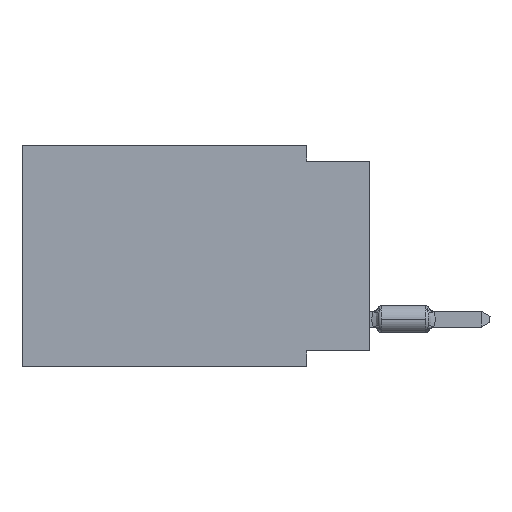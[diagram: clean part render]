
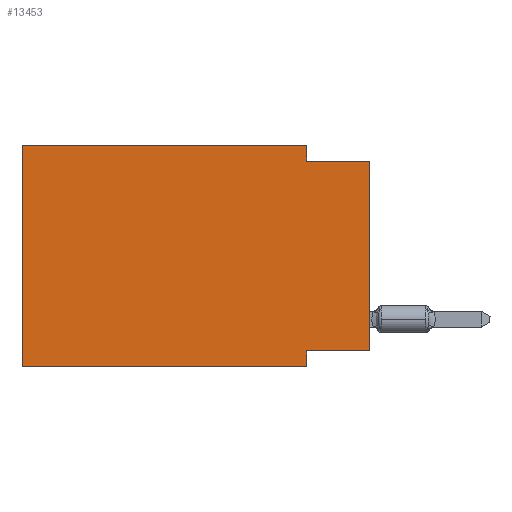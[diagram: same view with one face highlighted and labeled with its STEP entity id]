
A CAD part, left-side view. The second image highlights one B-rep face of the part: STEP entity #13453.
In plain terms, the highlighted planar face has unit normal (-1, 0, 0).
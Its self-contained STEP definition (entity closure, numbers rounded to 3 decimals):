
#489 = VERTEX_POINT ( 'NONE', #13293 ) ;
#593 = CARTESIAN_POINT ( 'NONE',  ( 0., 0., -8.255 ) ) ;
#1355 = VERTEX_POINT ( 'NONE', #31852 ) ;
#1724 = ORIENTED_EDGE ( 'NONE', *, *, #13110, .F. ) ;
#1796 = VECTOR ( 'NONE', #28328, 1000. ) ;
#2309 = ORIENTED_EDGE ( 'NONE', *, *, #19453, .T. ) ;
#2526 = EDGE_CURVE ( 'NONE', #1355, #23772, #24525, .T. ) ;
#3604 = ORIENTED_EDGE ( 'NONE', *, *, #8914, .F. ) ;
#4480 = VERTEX_POINT ( 'NONE', #32439 ) ;
#5051 = CARTESIAN_POINT ( 'NONE',  ( 0., 2.54, 0. ) ) ;
#7102 = EDGE_CURVE ( 'NONE', #22175, #12407, #18686, .T. ) ;
#7881 = EDGE_CURVE ( 'NONE', #4480, #12407, #21064, .T. ) ;
#8309 = DIRECTION ( 'NONE',  ( 0., 1., 0. ) ) ;
#8352 = CARTESIAN_POINT ( 'NONE',  ( 0., 13.97, -8.89 ) ) ;
#8555 = DIRECTION ( 'NONE',  ( 0., -1., 0. ) ) ;
#8914 = EDGE_CURVE ( 'NONE', #23772, #32596, #12694, .T. ) ;
#9343 = CARTESIAN_POINT ( 'NONE',  ( 0., 13.97, 0. ) ) ;
#9598 = EDGE_CURVE ( 'NONE', #29457, #22175, #11392, .T. ) ;
#10066 = CARTESIAN_POINT ( 'NONE',  ( 0., 0., 0. ) ) ;
#11025 = VECTOR ( 'NONE', #35230, 1000. ) ;
#11277 = CARTESIAN_POINT ( 'NONE',  ( 0., 0., -0.635 ) ) ;
#11392 = LINE ( 'NONE', #33937, #20119 ) ;
#11444 = VECTOR ( 'NONE', #38327, 1000. ) ;
#12407 = VERTEX_POINT ( 'NONE', #21204 ) ;
#12504 = CARTESIAN_POINT ( 'NONE',  ( 0., 2.54, -8.255 ) ) ;
#12694 = LINE ( 'NONE', #25207, #11025 ) ;
#13057 = CARTESIAN_POINT ( 'NONE',  ( 0., 2.54, -0.635 ) ) ;
#13091 = CARTESIAN_POINT ( 'NONE',  ( 0., 13.97, 0. ) ) ;
#13110 = EDGE_CURVE ( 'NONE', #32596, #489, #29722, .T. ) ;
#13293 = CARTESIAN_POINT ( 'NONE',  ( 0., 0., -0.635 ) ) ;
#13453 = ADVANCED_FACE ( 'NONE', ( #39485 ), #13475, .F. ) ;
#13475 = PLANE ( 'NONE',  #29024 ) ;
#14443 = CARTESIAN_POINT ( 'NONE',  ( 0., 13.97, 0. ) ) ;
#16191 = EDGE_CURVE ( 'NONE', #4480, #1355, #35645, .T. ) ;
#18172 = ORIENTED_EDGE ( 'NONE', *, *, #7102, .F. ) ;
#18686 = LINE ( 'NONE', #31198, #1796 ) ;
#19190 = EDGE_LOOP ( 'NONE', ( #2309, #1724, #3604, #34120, #21027, #36802, #18172, #26099 ) ) ;
#19453 = EDGE_CURVE ( 'NONE', #29457, #489, #28117, .T. ) ;
#20119 = VECTOR ( 'NONE', #8309, 1000. ) ;
#21027 = ORIENTED_EDGE ( 'NONE', *, *, #16191, .F. ) ;
#21064 = LINE ( 'NONE', #8352, #31911 ) ;
#21204 = CARTESIAN_POINT ( 'NONE',  ( 0., 2.54, -8.89 ) ) ;
#22175 = VERTEX_POINT ( 'NONE', #12504 ) ;
#22568 = DIRECTION ( 'NONE',  ( 0., 0., 1. ) ) ;
#23772 = VERTEX_POINT ( 'NONE', #5051 ) ;
#24081 = DIRECTION ( 'NONE',  ( 1., 0., 0. ) ) ;
#24525 = LINE ( 'NONE', #9343, #34061 ) ;
#25207 = CARTESIAN_POINT ( 'NONE',  ( 0., 2.54, 0. ) ) ;
#26099 = ORIENTED_EDGE ( 'NONE', *, *, #9598, .F. ) ;
#28117 = LINE ( 'NONE', #10066, #31138 ) ;
#28328 = DIRECTION ( 'NONE',  ( 0., 0., -1. ) ) ;
#29024 = AXIS2_PLACEMENT_3D ( 'NONE', #14443, #24081, #33522 ) ;
#29457 = VERTEX_POINT ( 'NONE', #593 ) ;
#29722 = LINE ( 'NONE', #11277, #38852 ) ;
#31138 = VECTOR ( 'NONE', #22568, 1000. ) ;
#31198 = CARTESIAN_POINT ( 'NONE',  ( 0., 2.54, -8.89 ) ) ;
#31852 = CARTESIAN_POINT ( 'NONE',  ( 0., 13.97, 0. ) ) ;
#31911 = VECTOR ( 'NONE', #8555, 1000. ) ;
#32187 = DIRECTION ( 'NONE',  ( 0., -1., 0. ) ) ;
#32439 = CARTESIAN_POINT ( 'NONE',  ( 0., 13.97, -8.89 ) ) ;
#32596 = VERTEX_POINT ( 'NONE', #13057 ) ;
#33522 = DIRECTION ( 'NONE',  ( 0., 0., -1. ) ) ;
#33562 = DIRECTION ( 'NONE',  ( 0., -1., 0. ) ) ;
#33937 = CARTESIAN_POINT ( 'NONE',  ( 0., 0., -8.255 ) ) ;
#34061 = VECTOR ( 'NONE', #33562, 1000. ) ;
#34120 = ORIENTED_EDGE ( 'NONE', *, *, #2526, .F. ) ;
#35230 = DIRECTION ( 'NONE',  ( 0., 0., -1. ) ) ;
#35645 = LINE ( 'NONE', #13091, #11444 ) ;
#36802 = ORIENTED_EDGE ( 'NONE', *, *, #7881, .T. ) ;
#38327 = DIRECTION ( 'NONE',  ( 0., 0., 1. ) ) ;
#38852 = VECTOR ( 'NONE', #32187, 1000. ) ;
#39485 = FACE_OUTER_BOUND ( 'NONE', #19190, .T. ) ;
